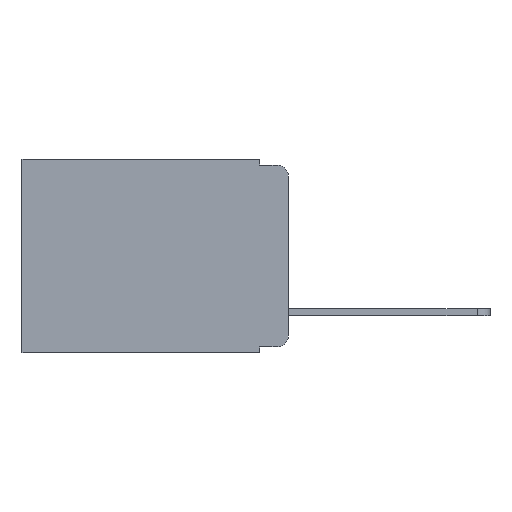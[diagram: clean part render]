
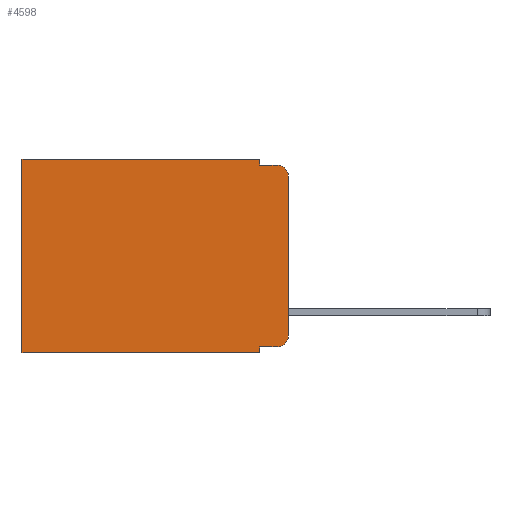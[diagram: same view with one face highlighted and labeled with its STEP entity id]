
A CAD part, left-side view. The second image highlights one B-rep face of the part: STEP entity #4598.
In plain terms, the highlighted planar face has unit normal (-1, 0, 0).
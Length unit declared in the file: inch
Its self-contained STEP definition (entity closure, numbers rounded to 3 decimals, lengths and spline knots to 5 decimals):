
#138 = EDGE_CURVE ( 'NONE', #13111, #20812, #20273, .T. ) ;
#311 = CARTESIAN_POINT ( 'NONE',  ( 0.298, 0., -0.03 ) ) ;
#756 = CARTESIAN_POINT ( 'NONE',  ( 0.298, 0.051, 0. ) ) ;
#854 = CARTESIAN_POINT ( 'NONE',  ( 0.298, 0.02, -0.01 ) ) ;
#1920 = EDGE_CURVE ( 'NONE', #18776, #17060, #17691, .T. ) ;
#2104 = ORIENTED_EDGE ( 'NONE', *, *, #17397, .F. ) ;
#2120 = FACE_OUTER_BOUND ( 'NONE', #4776, .T. ) ;
#2148 = VERTEX_POINT ( 'NONE', #8576 ) ;
#2295 = ORIENTED_EDGE ( 'NONE', *, *, #10810, .T. ) ;
#3492 = CARTESIAN_POINT ( 'NONE',  ( 0.298, 0.051, -0.01 ) ) ;
#3629 = ORIENTED_EDGE ( 'NONE', *, *, #138, .F. ) ;
#3674 = LINE ( 'NONE', #19414, #7627 ) ;
#4056 = ORIENTED_EDGE ( 'NONE', *, *, #14155, .F. ) ;
#4153 = CARTESIAN_POINT ( 'NONE',  ( 0.298, 0.02, -0.313 ) ) ;
#4598 = ADVANCED_FACE ( 'NONE', ( #2120 ), #19729, .F. ) ;
#4776 = EDGE_LOOP ( 'NONE', ( #10865, #6691, #2104, #3629, #2295, #9518, #4056, #6750, #6770, #4989 ) ) ;
#4989 = ORIENTED_EDGE ( 'NONE', *, *, #8067, .T. ) ;
#5044 = CIRCLE ( 'NONE', #21511, 0.02 ) ;
#5463 = VECTOR ( 'NONE', #7421, 39.37008 ) ;
#5749 = CARTESIAN_POINT ( 'NONE',  ( 0.298, 0.051, -0.333 ) ) ;
#5776 = AXIS2_PLACEMENT_3D ( 'NONE', #15799, #6123, #17434 ) ;
#5877 = DIRECTION ( 'NONE',  ( 0., 0., -1. ) ) ;
#5977 = LINE ( 'NONE', #12323, #14093 ) ;
#6123 = DIRECTION ( 'NONE',  ( -1., 0., 0. ) ) ;
#6691 = ORIENTED_EDGE ( 'NONE', *, *, #1920, .T. ) ;
#6750 = ORIENTED_EDGE ( 'NONE', *, *, #9482, .F. ) ;
#6770 = ORIENTED_EDGE ( 'NONE', *, *, #10283, .T. ) ;
#6917 = VECTOR ( 'NONE', #11148, 39.37008 ) ;
#7382 = VECTOR ( 'NONE', #15071, 39.37008 ) ;
#7421 = DIRECTION ( 'NONE',  ( 0., -1., 0. ) ) ;
#7627 = VECTOR ( 'NONE', #9787, 39.37008 ) ;
#7733 = LINE ( 'NONE', #11786, #15800 ) ;
#8067 = EDGE_CURVE ( 'NONE', #17976, #19843, #5044, .T. ) ;
#8576 = CARTESIAN_POINT ( 'NONE',  ( 0.298, 0.473, 0. ) ) ;
#8687 = CARTESIAN_POINT ( 'NONE',  ( 0.298, 0., 0. ) ) ;
#9482 = EDGE_CURVE ( 'NONE', #16586, #21319, #21145, .T. ) ;
#9518 = ORIENTED_EDGE ( 'NONE', *, *, #10541, .T. ) ;
#9787 = DIRECTION ( 'NONE',  ( 0., 0., -1. ) ) ;
#10152 = DIRECTION ( 'NONE',  ( 0., 0., -1. ) ) ;
#10283 = EDGE_CURVE ( 'NONE', #16586, #17976, #18403, .T. ) ;
#10541 = EDGE_CURVE ( 'NONE', #2148, #19945, #3674, .T. ) ;
#10637 = CARTESIAN_POINT ( 'NONE',  ( 0.298, 0.051, 0. ) ) ;
#10810 = EDGE_CURVE ( 'NONE', #13111, #2148, #15438, .T. ) ;
#10865 = ORIENTED_EDGE ( 'NONE', *, *, #21278, .F. ) ;
#11148 = DIRECTION ( 'NONE',  ( 0., 0., -1. ) ) ;
#11502 = CARTESIAN_POINT ( 'NONE',  ( 0.298, 0., -0.313 ) ) ;
#11786 = CARTESIAN_POINT ( 'NONE',  ( 0.298, 0., -0.343 ) ) ;
#12323 = CARTESIAN_POINT ( 'NONE',  ( 0.298, 0., 0. ) ) ;
#13111 = VERTEX_POINT ( 'NONE', #20361 ) ;
#13311 = CARTESIAN_POINT ( 'NONE',  ( 0.298, 0., 0. ) ) ;
#13399 = DIRECTION ( 'NONE',  ( 0., 1., 0. ) ) ;
#13941 = DIRECTION ( 'NONE',  ( 0., 0., -1. ) ) ;
#14093 = VECTOR ( 'NONE', #13941, 39.37008 ) ;
#14155 = EDGE_CURVE ( 'NONE', #21319, #19945, #7733, .T. ) ;
#14186 = DIRECTION ( 'NONE',  ( 0., 0., -1. ) ) ;
#14787 = CARTESIAN_POINT ( 'NONE',  ( 0.298, 0.02, -0.333 ) ) ;
#15071 = DIRECTION ( 'NONE',  ( 0., 1., 0. ) ) ;
#15172 = AXIS2_PLACEMENT_3D ( 'NONE', #13311, #19797, #10152 ) ;
#15438 = LINE ( 'NONE', #8687, #7382 ) ;
#15566 = DIRECTION ( 'NONE',  ( -1., 0., 0. ) ) ;
#15601 = CARTESIAN_POINT ( 'NONE',  ( 0.298, 0.051, -0.343 ) ) ;
#15799 = CARTESIAN_POINT ( 'NONE',  ( 0.298, 0.02, -0.03 ) ) ;
#15800 = VECTOR ( 'NONE', #13399, 39.37008 ) ;
#16586 = VERTEX_POINT ( 'NONE', #20413 ) ;
#17060 = VERTEX_POINT ( 'NONE', #854 ) ;
#17262 = VECTOR ( 'NONE', #18368, 39.37008 ) ;
#17397 = EDGE_CURVE ( 'NONE', #20812, #17060, #21507, .T. ) ;
#17434 = DIRECTION ( 'NONE',  ( 0., 0., -1. ) ) ;
#17617 = CARTESIAN_POINT ( 'NONE',  ( 0.298, 0.051, -0.01 ) ) ;
#17691 = CIRCLE ( 'NONE', #5776, 0.02 ) ;
#17976 = VERTEX_POINT ( 'NONE', #14787 ) ;
#18368 = DIRECTION ( 'NONE',  ( 0., -1., 0. ) ) ;
#18403 = LINE ( 'NONE', #5749, #5463 ) ;
#18776 = VERTEX_POINT ( 'NONE', #311 ) ;
#19414 = CARTESIAN_POINT ( 'NONE',  ( 0.298, 0.473, 0. ) ) ;
#19729 = PLANE ( 'NONE',  #15172 ) ;
#19797 = DIRECTION ( 'NONE',  ( 1., 0., 0. ) ) ;
#19843 = VERTEX_POINT ( 'NONE', #11502 ) ;
#19945 = VERTEX_POINT ( 'NONE', #21344 ) ;
#20273 = LINE ( 'NONE', #10637, #6917 ) ;
#20361 = CARTESIAN_POINT ( 'NONE',  ( 0.298, 0.051, 0. ) ) ;
#20413 = CARTESIAN_POINT ( 'NONE',  ( 0.298, 0.051, -0.333 ) ) ;
#20649 = VECTOR ( 'NONE', #14186, 39.37008 ) ;
#20812 = VERTEX_POINT ( 'NONE', #17617 ) ;
#21145 = LINE ( 'NONE', #756, #20649 ) ;
#21278 = EDGE_CURVE ( 'NONE', #18776, #19843, #5977, .T. ) ;
#21319 = VERTEX_POINT ( 'NONE', #15601 ) ;
#21344 = CARTESIAN_POINT ( 'NONE',  ( 0.298, 0.473, -0.343 ) ) ;
#21507 = LINE ( 'NONE', #3492, #17262 ) ;
#21511 = AXIS2_PLACEMENT_3D ( 'NONE', #4153, #15566, #5877 ) ;
